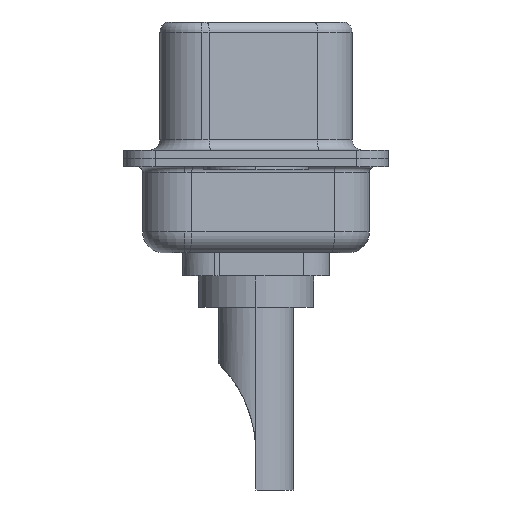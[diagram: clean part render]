
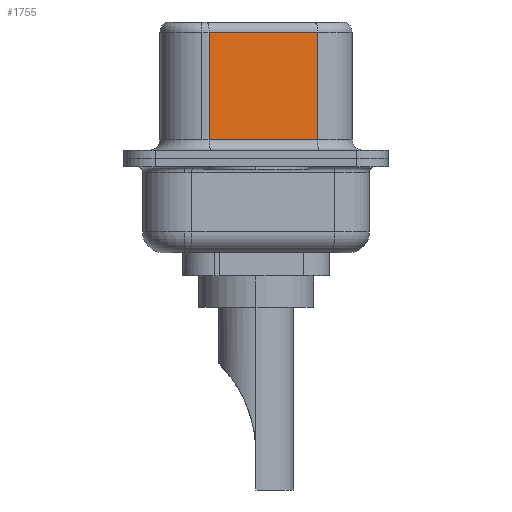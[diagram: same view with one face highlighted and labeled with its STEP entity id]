
A CAD part, left-side view. The second image highlights one B-rep face of the part: STEP entity #1755.
In plain terms, the highlighted planar face has unit normal (-0.985, -0.174, 0).
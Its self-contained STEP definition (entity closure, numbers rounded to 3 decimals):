
#180 = DIRECTION ( 'NONE',  ( 0., 0., -1. ) ) ;
#217 = PLANE ( 'NONE',  #4189 ) ;
#253 = ORIENTED_EDGE ( 'NONE', *, *, #3189, .T. ) ;
#350 = CARTESIAN_POINT ( 'NONE',  ( 4.585, -2.927, 6.52 ) ) ;
#595 = DIRECTION ( 'NONE',  ( 0.985, 0.174, 0. ) ) ;
#612 = VECTOR ( 'NONE', #180, 1000. ) ;
#639 = DIRECTION ( 'NONE',  ( -0.174, 0.985, 0. ) ) ;
#1755 = ADVANCED_FACE ( 'NONE', ( #6623 ), #217, .F. ) ;
#1849 = DIRECTION ( 'NONE',  ( 0., 0., -1. ) ) ;
#2099 = VERTEX_POINT ( 'NONE', #7507 ) ;
#2111 = CARTESIAN_POINT ( 'NONE',  ( 4.585, -2.927, 0.9 ) ) ;
#2406 = LINE ( 'NONE', #7770, #7686 ) ;
#2461 = VECTOR ( 'NONE', #8361, 1000. ) ;
#2641 = EDGE_CURVE ( 'NONE', #2099, #11468, #10780, .T. ) ;
#3189 = EDGE_CURVE ( 'NONE', #5977, #2099, #4175, .T. ) ;
#3538 = EDGE_CURVE ( 'NONE', #11468, #8098, #10021, .T. ) ;
#4175 = LINE ( 'NONE', #5925, #10356 ) ;
#4189 = AXIS2_PLACEMENT_3D ( 'NONE', #350, #595, #639 ) ;
#4404 = EDGE_LOOP ( 'NONE', ( #4609, #253, #5485, #9010 ) ) ;
#4485 = CARTESIAN_POINT ( 'NONE',  ( 3.675, 2.233, 0.9 ) ) ;
#4609 = ORIENTED_EDGE ( 'NONE', *, *, #6872, .F. ) ;
#4713 = CARTESIAN_POINT ( 'NONE',  ( 3.675, 2.233, 6.52 ) ) ;
#5485 = ORIENTED_EDGE ( 'NONE', *, *, #2641, .T. ) ;
#5646 = CARTESIAN_POINT ( 'NONE',  ( 4.585, -2.927, 6.02 ) ) ;
#5925 = CARTESIAN_POINT ( 'NONE',  ( 4.585, -2.927, 6.02 ) ) ;
#5977 = VERTEX_POINT ( 'NONE', #5646 ) ;
#6623 = FACE_OUTER_BOUND ( 'NONE', #4404, .T. ) ;
#6872 = EDGE_CURVE ( 'NONE', #5977, #8098, #2406, .T. ) ;
#7507 = CARTESIAN_POINT ( 'NONE',  ( 3.675, 2.233, 6.02 ) ) ;
#7573 = DIRECTION ( 'NONE',  ( -0.174, 0.985, 0. ) ) ;
#7686 = VECTOR ( 'NONE', #1849, 1000. ) ;
#7770 = CARTESIAN_POINT ( 'NONE',  ( 4.585, -2.927, 6.52 ) ) ;
#8098 = VERTEX_POINT ( 'NONE', #2111 ) ;
#8361 = DIRECTION ( 'NONE',  ( 0.174, -0.985, 0. ) ) ;
#8602 = CARTESIAN_POINT ( 'NONE',  ( 4.585, -2.927, 0.9 ) ) ;
#9010 = ORIENTED_EDGE ( 'NONE', *, *, #3538, .T. ) ;
#10021 = LINE ( 'NONE', #8602, #2461 ) ;
#10356 = VECTOR ( 'NONE', #7573, 1000. ) ;
#10780 = LINE ( 'NONE', #4713, #612 ) ;
#11468 = VERTEX_POINT ( 'NONE', #4485 ) ;
